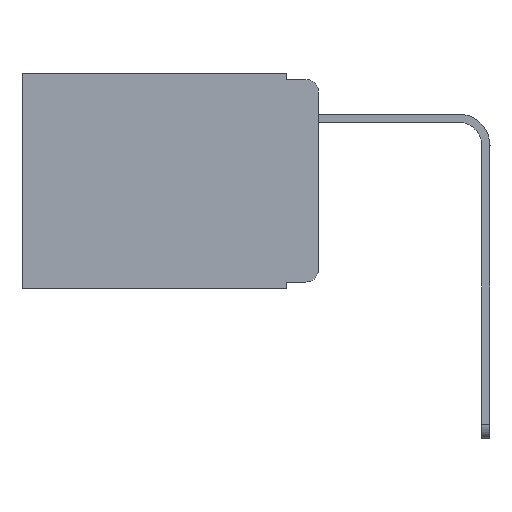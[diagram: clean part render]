
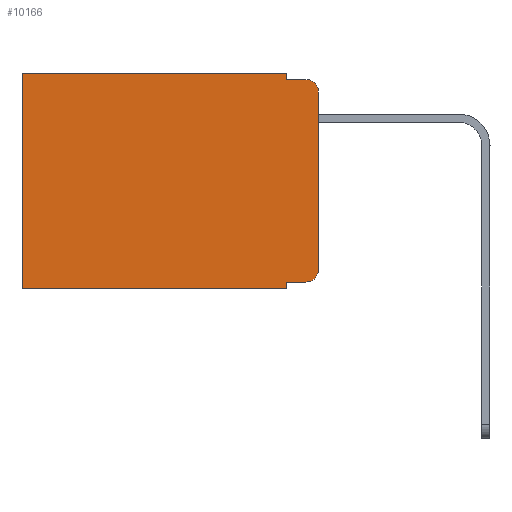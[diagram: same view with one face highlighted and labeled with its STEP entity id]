
A CAD part, left-side view. The second image highlights one B-rep face of the part: STEP entity #10166.
In plain terms, the highlighted planar face has unit normal (-1, 0, 0).
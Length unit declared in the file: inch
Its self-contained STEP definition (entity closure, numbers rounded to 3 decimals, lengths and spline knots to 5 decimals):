
#146 = DIRECTION ( 'NONE',  ( 1., 0., 0. ) ) ;
#348 = VECTOR ( 'NONE', #18605, 39.37008 ) ;
#442 = CARTESIAN_POINT ( 'NONE',  ( 0.298, 0.051, -0.01 ) ) ;
#795 = CARTESIAN_POINT ( 'NONE',  ( 0.298, 0.051, -0.333 ) ) ;
#854 = ORIENTED_EDGE ( 'NONE', *, *, #16270, .T. ) ;
#915 = VERTEX_POINT ( 'NONE', #1883 ) ;
#1095 = ORIENTED_EDGE ( 'NONE', *, *, #16458, .F. ) ;
#1602 = EDGE_CURVE ( 'NONE', #7657, #9802, #3989, .T. ) ;
#1883 = CARTESIAN_POINT ( 'NONE',  ( 0.298, 0.473, -0.343 ) ) ;
#3487 = ORIENTED_EDGE ( 'NONE', *, *, #15893, .F. ) ;
#3496 = CARTESIAN_POINT ( 'NONE',  ( 0.298, 0., 0. ) ) ;
#3972 = LINE ( 'NONE', #6612, #9853 ) ;
#3989 = LINE ( 'NONE', #16917, #348 ) ;
#4360 = CARTESIAN_POINT ( 'NONE',  ( 0.298, 0.051, -0.333 ) ) ;
#4487 = VERTEX_POINT ( 'NONE', #795 ) ;
#4648 = ORIENTED_EDGE ( 'NONE', *, *, #15007, .T. ) ;
#4892 = VECTOR ( 'NONE', #16874, 39.37008 ) ;
#4901 = EDGE_CURVE ( 'NONE', #4487, #5716, #12118, .T. ) ;
#5013 = DIRECTION ( 'NONE',  ( 0., 0., -1. ) ) ;
#5289 = AXIS2_PLACEMENT_3D ( 'NONE', #5519, #13937, #5433 ) ;
#5433 = DIRECTION ( 'NONE',  ( 0., 0., -1. ) ) ;
#5468 = DIRECTION ( 'NONE',  ( 0., -1., 0. ) ) ;
#5519 = CARTESIAN_POINT ( 'NONE',  ( 0.298, 0.02, -0.03 ) ) ;
#5716 = VERTEX_POINT ( 'NONE', #14525 ) ;
#6018 = VECTOR ( 'NONE', #18566, 39.37008 ) ;
#6612 = CARTESIAN_POINT ( 'NONE',  ( 0.298, 0.473, 0. ) ) ;
#6864 = CARTESIAN_POINT ( 'NONE',  ( 0.298, 0., 0. ) ) ;
#7011 = EDGE_CURVE ( 'NONE', #16183, #17276, #12947, .T. ) ;
#7106 = EDGE_CURVE ( 'NONE', #10710, #9802, #8427, .T. ) ;
#7135 = DIRECTION ( 'NONE',  ( -1., 0., 0. ) ) ;
#7211 = DIRECTION ( 'NONE',  ( 0., 0., -1. ) ) ;
#7223 = PLANE ( 'NONE',  #8806 ) ;
#7273 = ORIENTED_EDGE ( 'NONE', *, *, #7106, .T. ) ;
#7519 = CARTESIAN_POINT ( 'NONE',  ( 0.298, 0., -0.313 ) ) ;
#7657 = VERTEX_POINT ( 'NONE', #13893 ) ;
#7689 = CARTESIAN_POINT ( 'NONE',  ( 0.298, 0.473, 0. ) ) ;
#7758 = CARTESIAN_POINT ( 'NONE',  ( 0.298, 0., -0.343 ) ) ;
#7962 = LINE ( 'NONE', #3496, #4892 ) ;
#8124 = VECTOR ( 'NONE', #16328, 39.37008 ) ;
#8427 = CIRCLE ( 'NONE', #16418, 0.02 ) ;
#8551 = FACE_OUTER_BOUND ( 'NONE', #10265, .T. ) ;
#8806 = AXIS2_PLACEMENT_3D ( 'NONE', #6864, #146, #5013 ) ;
#8828 = CARTESIAN_POINT ( 'NONE',  ( 0.298, 0.02, -0.313 ) ) ;
#9802 = VERTEX_POINT ( 'NONE', #7519 ) ;
#9853 = VECTOR ( 'NONE', #18424, 39.37008 ) ;
#10166 = ADVANCED_FACE ( 'NONE', ( #8551 ), #7223, .F. ) ;
#10265 = EDGE_LOOP ( 'NONE', ( #12566, #4648, #1095, #12045, #21831, #12935, #3487, #17629, #854, #7273 ) ) ;
#10327 = CIRCLE ( 'NONE', #5289, 0.02 ) ;
#10710 = VERTEX_POINT ( 'NONE', #12507 ) ;
#11564 = LINE ( 'NONE', #4360, #12093 ) ;
#11846 = VECTOR ( 'NONE', #20273, 39.37008 ) ;
#12045 = ORIENTED_EDGE ( 'NONE', *, *, #7011, .F. ) ;
#12093 = VECTOR ( 'NONE', #5468, 39.37008 ) ;
#12118 = LINE ( 'NONE', #16880, #11846 ) ;
#12145 = EDGE_CURVE ( 'NONE', #15840, #915, #3972, .T. ) ;
#12179 = VECTOR ( 'NONE', #13727, 39.37008 ) ;
#12391 = EDGE_CURVE ( 'NONE', #16183, #15840, #7962, .T. ) ;
#12507 = CARTESIAN_POINT ( 'NONE',  ( 0.298, 0.02, -0.333 ) ) ;
#12566 = ORIENTED_EDGE ( 'NONE', *, *, #1602, .F. ) ;
#12935 = ORIENTED_EDGE ( 'NONE', *, *, #12145, .T. ) ;
#12947 = LINE ( 'NONE', #16967, #12179 ) ;
#13727 = DIRECTION ( 'NONE',  ( 0., 0., -1. ) ) ;
#13893 = CARTESIAN_POINT ( 'NONE',  ( 0.298, 0., -0.03 ) ) ;
#13937 = DIRECTION ( 'NONE',  ( -1., 0., 0. ) ) ;
#14220 = LINE ( 'NONE', #16645, #6018 ) ;
#14525 = CARTESIAN_POINT ( 'NONE',  ( 0.298, 0.051, -0.343 ) ) ;
#15007 = EDGE_CURVE ( 'NONE', #7657, #16260, #10327, .T. ) ;
#15840 = VERTEX_POINT ( 'NONE', #7689 ) ;
#15893 = EDGE_CURVE ( 'NONE', #5716, #915, #19205, .T. ) ;
#16183 = VERTEX_POINT ( 'NONE', #19080 ) ;
#16260 = VERTEX_POINT ( 'NONE', #17261 ) ;
#16270 = EDGE_CURVE ( 'NONE', #4487, #10710, #11564, .T. ) ;
#16328 = DIRECTION ( 'NONE',  ( 0., 1., 0. ) ) ;
#16418 = AXIS2_PLACEMENT_3D ( 'NONE', #8828, #7135, #7211 ) ;
#16458 = EDGE_CURVE ( 'NONE', #17276, #16260, #14220, .T. ) ;
#16645 = CARTESIAN_POINT ( 'NONE',  ( 0.298, 0.051, -0.01 ) ) ;
#16874 = DIRECTION ( 'NONE',  ( 0., 1., 0. ) ) ;
#16880 = CARTESIAN_POINT ( 'NONE',  ( 0.298, 0.051, 0. ) ) ;
#16917 = CARTESIAN_POINT ( 'NONE',  ( 0.298, 0., 0. ) ) ;
#16967 = CARTESIAN_POINT ( 'NONE',  ( 0.298, 0.051, 0. ) ) ;
#17261 = CARTESIAN_POINT ( 'NONE',  ( 0.298, 0.02, -0.01 ) ) ;
#17276 = VERTEX_POINT ( 'NONE', #442 ) ;
#17629 = ORIENTED_EDGE ( 'NONE', *, *, #4901, .F. ) ;
#18424 = DIRECTION ( 'NONE',  ( 0., 0., -1. ) ) ;
#18566 = DIRECTION ( 'NONE',  ( 0., -1., 0. ) ) ;
#18605 = DIRECTION ( 'NONE',  ( 0., 0., -1. ) ) ;
#19080 = CARTESIAN_POINT ( 'NONE',  ( 0.298, 0.051, 0. ) ) ;
#19205 = LINE ( 'NONE', #7758, #8124 ) ;
#20273 = DIRECTION ( 'NONE',  ( 0., 0., -1. ) ) ;
#21831 = ORIENTED_EDGE ( 'NONE', *, *, #12391, .T. ) ;
